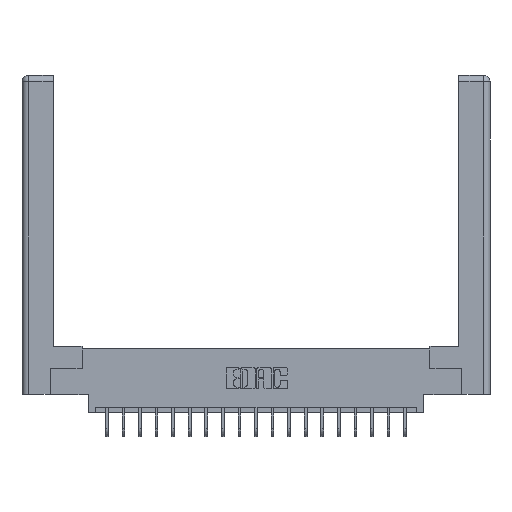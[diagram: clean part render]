
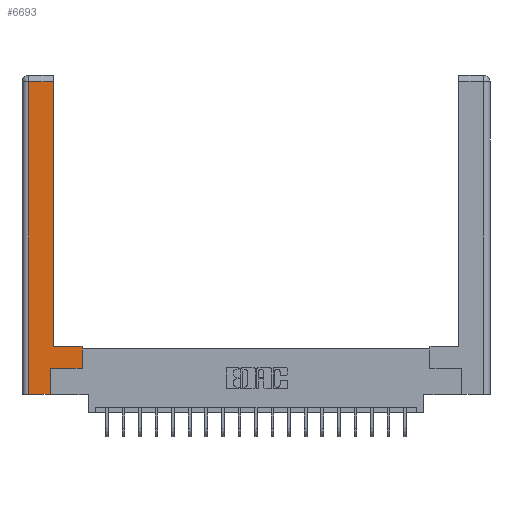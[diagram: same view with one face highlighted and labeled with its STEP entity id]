
A CAD part, top view. The second image highlights one B-rep face of the part: STEP entity #6693.
In plain terms, the highlighted planar face has unit normal (0, 0, 1).
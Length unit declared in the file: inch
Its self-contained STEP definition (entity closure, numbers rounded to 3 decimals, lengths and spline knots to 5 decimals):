
#32 = PLANE ( 'NONE',  #9769 ) ;
#121 = DIRECTION ( 'NONE',  ( -1., 0., 0. ) ) ;
#244 = EDGE_CURVE ( 'NONE', #19134, #19069, #17523, .T. ) ;
#1099 = VECTOR ( 'NONE', #15687, 39.37008 ) ;
#1522 = DIRECTION ( 'NONE',  ( 1., 0., 0. ) ) ;
#1688 = CARTESIAN_POINT ( 'NONE',  ( 0.565, 0.245, 0. ) ) ;
#1771 = CARTESIAN_POINT ( 'NONE',  ( 0.265, 0., 0. ) ) ;
#1865 = VECTOR ( 'NONE', #12233, 39.37008 ) ;
#2482 = EDGE_CURVE ( 'NONE', #6489, #21603, #17566, .T. ) ;
#2489 = LINE ( 'NONE', #17333, #14917 ) ;
#3027 = VERTEX_POINT ( 'NONE', #19411 ) ;
#3746 = ORIENTED_EDGE ( 'NONE', *, *, #244, .T. ) ;
#3837 = EDGE_CURVE ( 'NONE', #11793, #3027, #5115, .T. ) ;
#3926 = DIRECTION ( 'NONE',  ( -1., 0., 0. ) ) ;
#4420 = DIRECTION ( 'NONE',  ( 0., 1., 0. ) ) ;
#4426 = ORIENTED_EDGE ( 'NONE', *, *, #20680, .T. ) ;
#5115 = LINE ( 'NONE', #10453, #1099 ) ;
#5570 = VECTOR ( 'NONE', #4420, 39.37008 ) ;
#6263 = CARTESIAN_POINT ( 'NONE',  ( 0.265, 0., 0. ) ) ;
#6489 = VERTEX_POINT ( 'NONE', #7796 ) ;
#6693 = ADVANCED_FACE ( 'NONE', ( #18980 ), #32, .F. ) ;
#7085 = DIRECTION ( 'NONE',  ( 0., 0., -1. ) ) ;
#7405 = CARTESIAN_POINT ( 'NONE',  ( 0.295, 0.45, 0. ) ) ;
#7796 = CARTESIAN_POINT ( 'NONE',  ( 0.565, 0.45, 0. ) ) ;
#7950 = EDGE_CURVE ( 'NONE', #3027, #19134, #21249, .T. ) ;
#8432 = VECTOR ( 'NONE', #121, 39.37008 ) ;
#8585 = CARTESIAN_POINT ( 'NONE',  ( 0.0615, 2.94, 0. ) ) ;
#8812 = ORIENTED_EDGE ( 'NONE', *, *, #7950, .T. ) ;
#9064 = CARTESIAN_POINT ( 'NONE',  ( 0.295, 2.94, 0. ) ) ;
#9186 = EDGE_CURVE ( 'NONE', #19069, #10052, #10188, .T. ) ;
#9728 = EDGE_CURVE ( 'NONE', #14234, #11793, #21988, .T. ) ;
#9769 = AXIS2_PLACEMENT_3D ( 'NONE', #20817, #7085, #3926 ) ;
#9858 = ORIENTED_EDGE ( 'NONE', *, *, #15617, .T. ) ;
#10052 = VERTEX_POINT ( 'NONE', #1688 ) ;
#10188 = LINE ( 'NONE', #11760, #15323 ) ;
#10453 = CARTESIAN_POINT ( 'NONE',  ( 0.0615, 0., 0. ) ) ;
#10507 = CARTESIAN_POINT ( 'NONE',  ( 0.295, 0.45, 0. ) ) ;
#11734 = ORIENTED_EDGE ( 'NONE', *, *, #9186, .T. ) ;
#11760 = CARTESIAN_POINT ( 'NONE',  ( 0.565, 0.245, 0. ) ) ;
#11793 = VERTEX_POINT ( 'NONE', #8585 ) ;
#11805 = LINE ( 'NONE', #14693, #5570 ) ;
#12233 = DIRECTION ( 'NONE',  ( 1., 0., 0. ) ) ;
#12876 = VECTOR ( 'NONE', #18930, 39.37008 ) ;
#12993 = VECTOR ( 'NONE', #20639, 39.37008 ) ;
#13731 = ORIENTED_EDGE ( 'NONE', *, *, #9728, .T. ) ;
#14234 = VERTEX_POINT ( 'NONE', #9064 ) ;
#14693 = CARTESIAN_POINT ( 'NONE',  ( 0.295, 3., 0. ) ) ;
#14917 = VECTOR ( 'NONE', #17260, 39.37008 ) ;
#15323 = VECTOR ( 'NONE', #1522, 39.37008 ) ;
#15617 = EDGE_CURVE ( 'NONE', #21603, #14234, #11805, .T. ) ;
#15687 = DIRECTION ( 'NONE',  ( 0., -1., 0. ) ) ;
#16583 = EDGE_LOOP ( 'NONE', ( #9858, #13731, #22251, #8812, #3746, #11734, #4426, #22139 ) ) ;
#16837 = CARTESIAN_POINT ( 'NONE',  ( 0.265, 0.245, 0. ) ) ;
#17260 = DIRECTION ( 'NONE',  ( 0., 1., 0. ) ) ;
#17333 = CARTESIAN_POINT ( 'NONE',  ( 0.565, 0.45, 0. ) ) ;
#17523 = LINE ( 'NONE', #16837, #12993 ) ;
#17566 = LINE ( 'NONE', #10507, #8432 ) ;
#18313 = CARTESIAN_POINT ( 'NONE',  ( 0.265, 0.245, 0. ) ) ;
#18930 = DIRECTION ( 'NONE',  ( -1., 0., 0. ) ) ;
#18980 = FACE_OUTER_BOUND ( 'NONE', #16583, .T. ) ;
#19069 = VERTEX_POINT ( 'NONE', #18313 ) ;
#19134 = VERTEX_POINT ( 'NONE', #6263 ) ;
#19411 = CARTESIAN_POINT ( 'NONE',  ( 0.0615, 0., 0. ) ) ;
#20639 = DIRECTION ( 'NONE',  ( 0., 1., 0. ) ) ;
#20680 = EDGE_CURVE ( 'NONE', #10052, #6489, #2489, .T. ) ;
#20817 = CARTESIAN_POINT ( 'NONE',  ( 0., 0., 0. ) ) ;
#20890 = CARTESIAN_POINT ( 'NONE',  ( 0.0615, 2.94, 0. ) ) ;
#21249 = LINE ( 'NONE', #1771, #1865 ) ;
#21603 = VERTEX_POINT ( 'NONE', #7405 ) ;
#21988 = LINE ( 'NONE', #20890, #12876 ) ;
#22139 = ORIENTED_EDGE ( 'NONE', *, *, #2482, .T. ) ;
#22251 = ORIENTED_EDGE ( 'NONE', *, *, #3837, .T. ) ;
